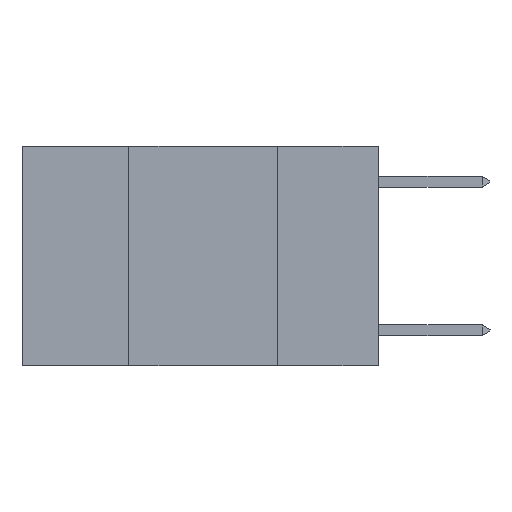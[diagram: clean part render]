
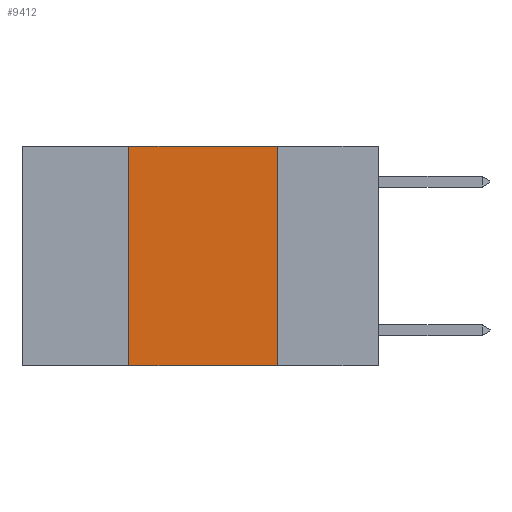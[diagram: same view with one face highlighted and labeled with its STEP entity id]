
A CAD part, left-side view. The second image highlights one B-rep face of the part: STEP entity #9412.
In plain terms, the highlighted planar face has unit normal (-1, 0, 0).
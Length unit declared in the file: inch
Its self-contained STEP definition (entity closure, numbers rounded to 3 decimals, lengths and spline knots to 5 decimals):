
#1925 = AXIS2_PLACEMENT_3D ( 'NONE', #20082, #24812, #10564 ) ;
#2637 = ORIENTED_EDGE ( 'NONE', *, *, #12770, .F. ) ;
#3844 = VECTOR ( 'NONE', #18639, 39.37008 ) ;
#5404 = CARTESIAN_POINT ( 'NONE',  ( 0., 0.17, 0. ) ) ;
#7299 = DIRECTION ( 'NONE',  ( 0., 0., 1. ) ) ;
#7768 = DIRECTION ( 'NONE',  ( 0., 0., -1. ) ) ;
#8062 = LINE ( 'NONE', #5404, #19996 ) ;
#8534 = EDGE_CURVE ( 'NONE', #11910, #18207, #18691, .T. ) ;
#8980 = ORIENTED_EDGE ( 'NONE', *, *, #27091, .F. ) ;
#9412 = ADVANCED_FACE ( 'NONE', ( #25656 ), #22458, .F. ) ;
#10449 = VERTEX_POINT ( 'NONE', #28674 ) ;
#10564 = DIRECTION ( 'NONE',  ( 0., 0., -1. ) ) ;
#11910 = VERTEX_POINT ( 'NONE', #18765 ) ;
#12487 = CARTESIAN_POINT ( 'NONE',  ( 0., 0.17, 0. ) ) ;
#12770 = EDGE_CURVE ( 'NONE', #18207, #25172, #8062, .T. ) ;
#14385 = CARTESIAN_POINT ( 'NONE',  ( 0., 0.42, 0. ) ) ;
#16246 = CARTESIAN_POINT ( 'NONE',  ( 0., 0.6, -0.37 ) ) ;
#18207 = VERTEX_POINT ( 'NONE', #12487 ) ;
#18639 = DIRECTION ( 'NONE',  ( 0., -1., 0. ) ) ;
#18691 = LINE ( 'NONE', #26506, #24219 ) ;
#18765 = CARTESIAN_POINT ( 'NONE',  ( 0., 0.42, 0. ) ) ;
#19996 = VECTOR ( 'NONE', #7768, 39.37008 ) ;
#20082 = CARTESIAN_POINT ( 'NONE',  ( 0., 0.6, 0. ) ) ;
#21680 = ORIENTED_EDGE ( 'NONE', *, *, #8534, .F. ) ;
#22458 = PLANE ( 'NONE',  #1925 ) ;
#22842 = LINE ( 'NONE', #16246, #3844 ) ;
#23149 = ORIENTED_EDGE ( 'NONE', *, *, #25510, .T. ) ;
#24219 = VECTOR ( 'NONE', #28874, 39.37008 ) ;
#24250 = LINE ( 'NONE', #14385, #29786 ) ;
#24812 = DIRECTION ( 'NONE',  ( 1., 0., 0. ) ) ;
#25172 = VERTEX_POINT ( 'NONE', #29177 ) ;
#25510 = EDGE_CURVE ( 'NONE', #10449, #25172, #22842, .T. ) ;
#25656 = FACE_OUTER_BOUND ( 'NONE', #26405, .T. ) ;
#26405 = EDGE_LOOP ( 'NONE', ( #2637, #21680, #8980, #23149 ) ) ;
#26506 = CARTESIAN_POINT ( 'NONE',  ( 0., 0.6, 0. ) ) ;
#27091 = EDGE_CURVE ( 'NONE', #10449, #11910, #24250, .T. ) ;
#28674 = CARTESIAN_POINT ( 'NONE',  ( 0., 0.42, -0.37 ) ) ;
#28874 = DIRECTION ( 'NONE',  ( 0., -1., 0. ) ) ;
#29177 = CARTESIAN_POINT ( 'NONE',  ( 0., 0.17, -0.37 ) ) ;
#29786 = VECTOR ( 'NONE', #7299, 39.37008 ) ;
